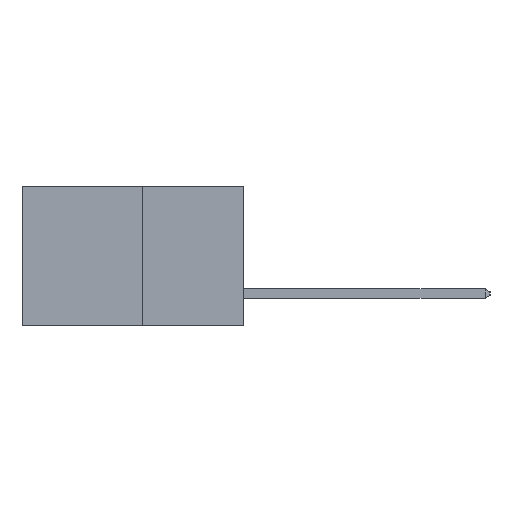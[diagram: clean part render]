
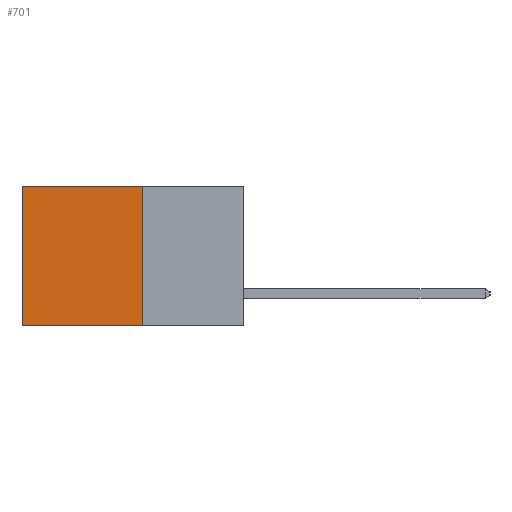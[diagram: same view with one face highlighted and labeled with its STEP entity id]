
A CAD part, left-side view. The second image highlights one B-rep face of the part: STEP entity #701.
In plain terms, the highlighted planar face has unit normal (-1, 0, 0).
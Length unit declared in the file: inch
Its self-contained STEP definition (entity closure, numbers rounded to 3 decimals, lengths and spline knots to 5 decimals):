
#15 = AXIS2_PLACEMENT_3D ( 'NONE', #8979, #2221, #6671 ) ;
#35 = VECTOR ( 'NONE', #331, 39.37008 ) ;
#331 = DIRECTION ( 'NONE',  ( 0., 0., -1. ) ) ;
#514 = VERTEX_POINT ( 'NONE', #3217 ) ;
#701 = ADVANCED_FACE ( 'NONE', ( #5743 ), #7751, .F. ) ;
#1102 = LINE ( 'NONE', #4104, #5095 ) ;
#2221 = DIRECTION ( 'NONE',  ( 1., 0., 0. ) ) ;
#2561 = LINE ( 'NONE', #5156, #35 ) ;
#3217 = CARTESIAN_POINT ( 'NONE',  ( 0.277, 0.59, -0.37 ) ) ;
#3800 = ORIENTED_EDGE ( 'NONE', *, *, #4050, .F. ) ;
#4050 = EDGE_CURVE ( 'NONE', #5786, #514, #1102, .T. ) ;
#4104 = CARTESIAN_POINT ( 'NONE',  ( 0.277, 0.27, -0.37 ) ) ;
#4273 = VERTEX_POINT ( 'NONE', #8096 ) ;
#4323 = EDGE_CURVE ( 'NONE', #9746, #514, #8765, .T. ) ;
#4459 = DIRECTION ( 'NONE',  ( 0., 1., 0. ) ) ;
#4496 = EDGE_LOOP ( 'NONE', ( #8164, #3800, #5794, #5868 ) ) ;
#4691 = DIRECTION ( 'NONE',  ( 0., 1., 0. ) ) ;
#4984 = VECTOR ( 'NONE', #8902, 39.37008 ) ;
#5095 = VECTOR ( 'NONE', #4691, 39.37008 ) ;
#5156 = CARTESIAN_POINT ( 'NONE',  ( 0.277, 0.27, -0.37 ) ) ;
#5425 = VECTOR ( 'NONE', #4459, 39.37008 ) ;
#5656 = LINE ( 'NONE', #5951, #5425 ) ;
#5743 = FACE_OUTER_BOUND ( 'NONE', #4496, .T. ) ;
#5786 = VERTEX_POINT ( 'NONE', #7838 ) ;
#5794 = ORIENTED_EDGE ( 'NONE', *, *, #7786, .F. ) ;
#5868 = ORIENTED_EDGE ( 'NONE', *, *, #7901, .T. ) ;
#5951 = CARTESIAN_POINT ( 'NONE',  ( 0.277, 0.27, 0. ) ) ;
#6349 = CARTESIAN_POINT ( 'NONE',  ( 0.277, 0.59, 0. ) ) ;
#6671 = DIRECTION ( 'NONE',  ( 0., 0., -1. ) ) ;
#7751 = PLANE ( 'NONE',  #15 ) ;
#7786 = EDGE_CURVE ( 'NONE', #4273, #5786, #2561, .T. ) ;
#7838 = CARTESIAN_POINT ( 'NONE',  ( 0.277, 0.27, -0.37 ) ) ;
#7901 = EDGE_CURVE ( 'NONE', #4273, #9746, #5656, .T. ) ;
#8096 = CARTESIAN_POINT ( 'NONE',  ( 0.277, 0.27, 0. ) ) ;
#8164 = ORIENTED_EDGE ( 'NONE', *, *, #4323, .T. ) ;
#8307 = CARTESIAN_POINT ( 'NONE',  ( 0.277, 0.59, -0.37 ) ) ;
#8765 = LINE ( 'NONE', #8307, #4984 ) ;
#8902 = DIRECTION ( 'NONE',  ( 0., 0., -1. ) ) ;
#8979 = CARTESIAN_POINT ( 'NONE',  ( 0.277, 0.27, -0.37 ) ) ;
#9746 = VERTEX_POINT ( 'NONE', #6349 ) ;
